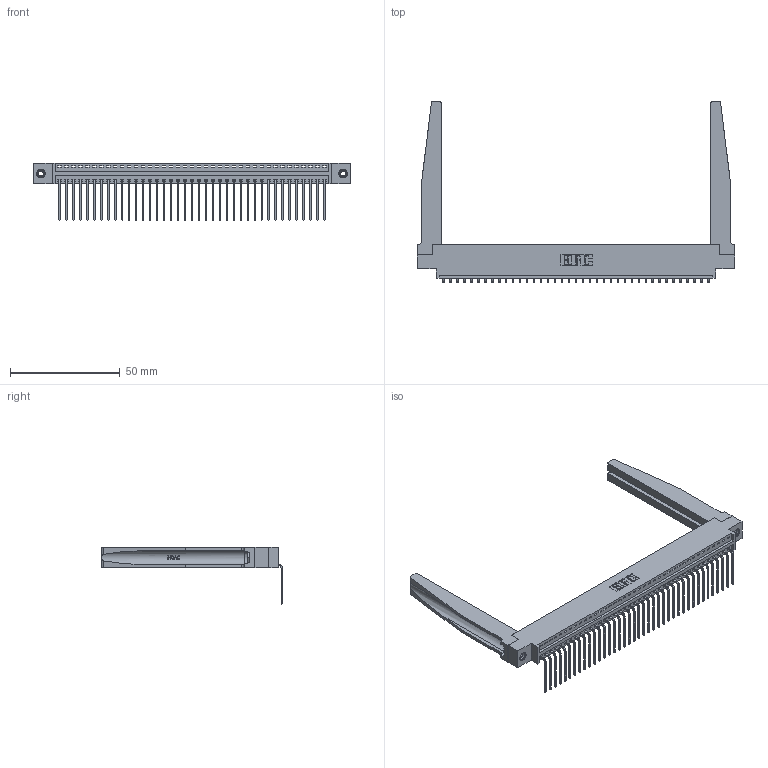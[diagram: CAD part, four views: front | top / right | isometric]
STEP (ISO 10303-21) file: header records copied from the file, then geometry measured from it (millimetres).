
FILE_DESCRIPTION (( 'STEP AP203' ), '1' );
FILE_NAME ('396-039-559-678.STEP', '2019-10-31T22:42:29', ( '' ), ( '' ), 'SwSTEP 2.0', 'SolidWorks 2016', '' );
FILE_SCHEMA (( 'CONFIG_CONTROL_DESIGN' ));
Length unit declared in the file: inch
Products named in the file (5): 346 Part_0.170 Offset - 0.156 Dia-TH; 345-292-001_558 559 Tail - 1; 346-220-078_345-220-078; 345-250-001_345-250-001-102; 396-039-559-678
Assembly tree (44 placements, depth 2):
  396-039-559-678
    346 Part_0.170 Offset - 0.156 Dia-TH
    345-292-001_558 559 Tail - 1  x39
    346-220-078_345-220-078  x2
    345-250-001_345-250-001-102  x2
Bounding box: 144.4 x 82.36 x 26.16 mm (x, y, z)
Volume: 20685.7 mm3; surface area: 24662.5 mm2
Topology: 44 solids, 44 shells, 2700 faces, 8047 edges, 5302 vertices
Faces by surface type: plane 1860, cylinder 788, bspline 36, cone 12, torus 4
Entity records: 29572 total; most frequent: CARTESIAN_POINT 5984, ORIENTED_EDGE 4846, DIRECTION 4267, EDGE_CURVE 2423, VECTOR 2041, LINE 2041, VERTEX_POINT 1608, AXIS2_PLACEMENT_3D 1113
